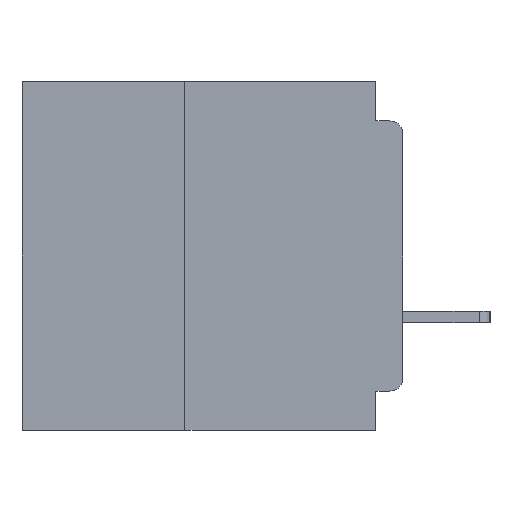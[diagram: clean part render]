
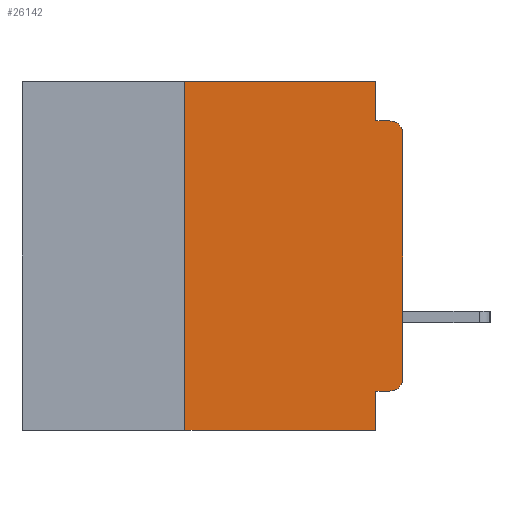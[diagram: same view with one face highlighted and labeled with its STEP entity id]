
A CAD part, left-side view. The second image highlights one B-rep face of the part: STEP entity #26142.
In plain terms, the highlighted planar face has unit normal (-1, 0, 0).
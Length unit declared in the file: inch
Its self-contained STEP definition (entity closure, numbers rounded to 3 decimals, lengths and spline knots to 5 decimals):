
#48 = VECTOR ( 'NONE', #30538, 39.37008 ) ;
#94 = PLANE ( 'NONE',  #31271 ) ;
#1480 = AXIS2_PLACEMENT_3D ( 'NONE', #35574, #16063, #38803 ) ;
#2174 = FACE_OUTER_BOUND ( 'NONE', #4836, .T. ) ;
#2770 = LINE ( 'NONE', #11788, #36438 ) ;
#3426 = DIRECTION ( 'NONE',  ( 1., 0., 0. ) ) ;
#3660 = DIRECTION ( 'NONE',  ( 0., -1., 0. ) ) ;
#4352 = VECTOR ( 'NONE', #3660, 39.37008 ) ;
#4716 = CARTESIAN_POINT ( 'NONE',  ( 0., 0.015, -0.06 ) ) ;
#4794 = ORIENTED_EDGE ( 'NONE', *, *, #24517, .T. ) ;
#4836 = EDGE_LOOP ( 'NONE', ( #36389, #22839, #37204, #28232, #32249, #9439, #4794, #17380, #15959, #4864 ) ) ;
#4864 = ORIENTED_EDGE ( 'NONE', *, *, #15367, .T. ) ;
#4918 = EDGE_CURVE ( 'NONE', #16365, #42012, #24932, .T. ) ;
#6526 = VECTOR ( 'NONE', #19474, 39.37008 ) ;
#6740 = LINE ( 'NONE', #16628, #40287 ) ;
#6935 = DIRECTION ( 'NONE',  ( 0., 0., -1. ) ) ;
#7511 = VERTEX_POINT ( 'NONE', #36337 ) ;
#7974 = DIRECTION ( 'NONE',  ( 0., 0., -1. ) ) ;
#8330 = VERTEX_POINT ( 'NONE', #27880 ) ;
#8399 = EDGE_CURVE ( 'NONE', #42012, #24789, #2770, .T. ) ;
#8788 = LINE ( 'NONE', #40112, #48 ) ;
#9439 = ORIENTED_EDGE ( 'NONE', *, *, #10722, .F. ) ;
#10722 = EDGE_CURVE ( 'NONE', #8330, #20512, #11783, .T. ) ;
#10931 = CARTESIAN_POINT ( 'NONE',  ( 0., 0.437, 0. ) ) ;
#11783 = LINE ( 'NONE', #41747, #28109 ) ;
#11788 = CARTESIAN_POINT ( 'NONE',  ( 0., 0.031, -0.4 ) ) ;
#13097 = CIRCLE ( 'NONE', #35307, 0.015 ) ;
#13158 = CARTESIAN_POINT ( 'NONE',  ( 0., 0.437, 0. ) ) ;
#15367 = EDGE_CURVE ( 'NONE', #16365, #23321, #38049, .T. ) ;
#15959 = ORIENTED_EDGE ( 'NONE', *, *, #4918, .F. ) ;
#16063 = DIRECTION ( 'NONE',  ( -1., 0., 0. ) ) ;
#16365 = VERTEX_POINT ( 'NONE', #34089 ) ;
#16628 = CARTESIAN_POINT ( 'NONE',  ( 0., 0.031, 0. ) ) ;
#17380 = ORIENTED_EDGE ( 'NONE', *, *, #8399, .F. ) ;
#19474 = DIRECTION ( 'NONE',  ( 0., 0., 1. ) ) ;
#19698 = CARTESIAN_POINT ( 'NONE',  ( 0., 0.031, 0. ) ) ;
#20512 = VERTEX_POINT ( 'NONE', #34640 ) ;
#21587 = VERTEX_POINT ( 'NONE', #27445 ) ;
#21716 = LINE ( 'NONE', #23266, #4352 ) ;
#21745 = DIRECTION ( 'NONE',  ( 0., 0., -1. ) ) ;
#22199 = EDGE_CURVE ( 'NONE', #7511, #33635, #13097, .T. ) ;
#22409 = DIRECTION ( 'NONE',  ( 0., 0., 1. ) ) ;
#22665 = EDGE_CURVE ( 'NONE', #21587, #33635, #21716, .T. ) ;
#22796 = EDGE_CURVE ( 'NONE', #20512, #36718, #32940, .T. ) ;
#22839 = ORIENTED_EDGE ( 'NONE', *, *, #22199, .T. ) ;
#23266 = CARTESIAN_POINT ( 'NONE',  ( 0., 0., -0.045 ) ) ;
#23321 = VERTEX_POINT ( 'NONE', #26473 ) ;
#24517 = EDGE_CURVE ( 'NONE', #8330, #24789, #8788, .T. ) ;
#24789 = VERTEX_POINT ( 'NONE', #25416 ) ;
#24932 = LINE ( 'NONE', #38795, #33573 ) ;
#25416 = CARTESIAN_POINT ( 'NONE',  ( 0., 0.031, -0.4 ) ) ;
#26142 = ADVANCED_FACE ( 'NONE', ( #2174 ), #94, .F. ) ;
#26286 = DIRECTION ( 'NONE',  ( 0., 0., -1. ) ) ;
#26473 = CARTESIAN_POINT ( 'NONE',  ( 0., 0., -0.34 ) ) ;
#27445 = CARTESIAN_POINT ( 'NONE',  ( 0., 0.031, -0.045 ) ) ;
#27534 = DIRECTION ( 'NONE',  ( -1., 0., 0. ) ) ;
#27880 = CARTESIAN_POINT ( 'NONE',  ( 0., 0.25, -0.4 ) ) ;
#28109 = VECTOR ( 'NONE', #22409, 39.37008 ) ;
#28232 = ORIENTED_EDGE ( 'NONE', *, *, #32253, .F. ) ;
#30538 = DIRECTION ( 'NONE',  ( 0., -1., 0. ) ) ;
#31271 = AXIS2_PLACEMENT_3D ( 'NONE', #13158, #3426, #26286 ) ;
#31533 = LINE ( 'NONE', #41397, #6526 ) ;
#32249 = ORIENTED_EDGE ( 'NONE', *, *, #22796, .F. ) ;
#32253 = EDGE_CURVE ( 'NONE', #36718, #21587, #6740, .T. ) ;
#32940 = LINE ( 'NONE', #10931, #40441 ) ;
#33573 = VECTOR ( 'NONE', #38757, 39.37008 ) ;
#33635 = VERTEX_POINT ( 'NONE', #39926 ) ;
#34089 = CARTESIAN_POINT ( 'NONE',  ( 0., 0.015, -0.355 ) ) ;
#34640 = CARTESIAN_POINT ( 'NONE',  ( 0., 0.25, 0. ) ) ;
#35307 = AXIS2_PLACEMENT_3D ( 'NONE', #4716, #27534, #7974 ) ;
#35574 = CARTESIAN_POINT ( 'NONE',  ( 0., 0.015, -0.34 ) ) ;
#36337 = CARTESIAN_POINT ( 'NONE',  ( 0., 0., -0.06 ) ) ;
#36389 = ORIENTED_EDGE ( 'NONE', *, *, #37763, .T. ) ;
#36438 = VECTOR ( 'NONE', #21745, 39.37008 ) ;
#36718 = VERTEX_POINT ( 'NONE', #19698 ) ;
#36989 = DIRECTION ( 'NONE',  ( 0., -1., 0. ) ) ;
#37204 = ORIENTED_EDGE ( 'NONE', *, *, #22665, .F. ) ;
#37763 = EDGE_CURVE ( 'NONE', #23321, #7511, #31533, .T. ) ;
#38049 = CIRCLE ( 'NONE', #1480, 0.015 ) ;
#38757 = DIRECTION ( 'NONE',  ( 0., 1., 0. ) ) ;
#38795 = CARTESIAN_POINT ( 'NONE',  ( 0., 0., -0.355 ) ) ;
#38803 = DIRECTION ( 'NONE',  ( 0., 0., -1. ) ) ;
#39926 = CARTESIAN_POINT ( 'NONE',  ( 0., 0.015, -0.045 ) ) ;
#40112 = CARTESIAN_POINT ( 'NONE',  ( 0., 0.437, -0.4 ) ) ;
#40287 = VECTOR ( 'NONE', #6935, 39.37008 ) ;
#40441 = VECTOR ( 'NONE', #36989, 39.37008 ) ;
#41397 = CARTESIAN_POINT ( 'NONE',  ( 0., 0., 0. ) ) ;
#41747 = CARTESIAN_POINT ( 'NONE',  ( 0., 0.25, -0.4 ) ) ;
#41812 = CARTESIAN_POINT ( 'NONE',  ( 0., 0.031, -0.355 ) ) ;
#42012 = VERTEX_POINT ( 'NONE', #41812 ) ;
